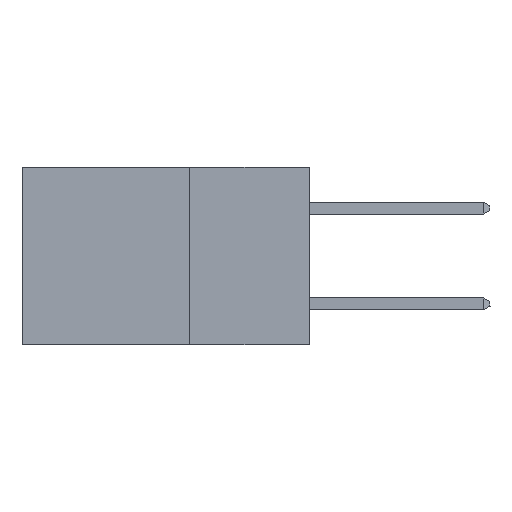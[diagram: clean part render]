
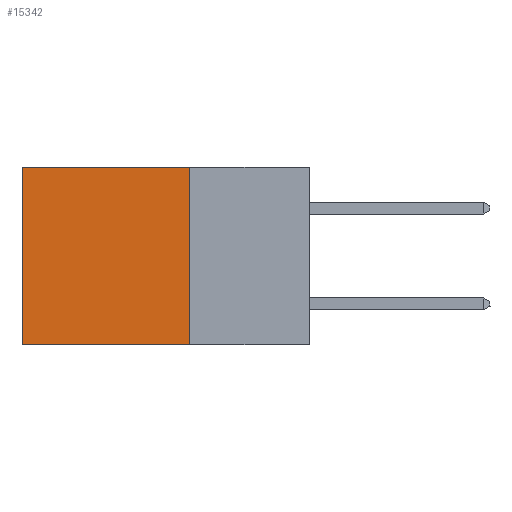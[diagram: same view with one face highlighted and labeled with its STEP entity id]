
A CAD part, left-side view. The second image highlights one B-rep face of the part: STEP entity #15342.
In plain terms, the highlighted planar face has unit normal (-1, 0, 0).
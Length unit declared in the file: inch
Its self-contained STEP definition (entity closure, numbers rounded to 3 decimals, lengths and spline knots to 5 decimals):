
#981 = EDGE_LOOP ( 'NONE', ( #32184, #5134, #12946, #16790 ) ) ;
#1453 = CARTESIAN_POINT ( 'NONE',  ( 0.2875, 0.25, 0. ) ) ;
#1958 = DIRECTION ( 'NONE',  ( 0., 1., 0. ) ) ;
#2166 = CARTESIAN_POINT ( 'NONE',  ( 0.2875, 0.6, 0. ) ) ;
#4519 = CARTESIAN_POINT ( 'NONE',  ( 0.2875, 0.25, -0.37 ) ) ;
#5134 = ORIENTED_EDGE ( 'NONE', *, *, #17647, .F. ) ;
#7228 = DIRECTION ( 'NONE',  ( 0., 1., 0. ) ) ;
#8086 = LINE ( 'NONE', #29395, #22522 ) ;
#8481 = CARTESIAN_POINT ( 'NONE',  ( 0.2875, 0.25, -0.37 ) ) ;
#9485 = DIRECTION ( 'NONE',  ( 1., 0., 0. ) ) ;
#9919 = VERTEX_POINT ( 'NONE', #8481 ) ;
#10377 = EDGE_CURVE ( 'NONE', #26459, #28459, #15561, .T. ) ;
#10738 = VECTOR ( 'NONE', #7228, 39.37008 ) ;
#12946 = ORIENTED_EDGE ( 'NONE', *, *, #13457, .F. ) ;
#13107 = CARTESIAN_POINT ( 'NONE',  ( 0.2875, 0.6, 0. ) ) ;
#13457 = EDGE_CURVE ( 'NONE', #22661, #9919, #8086, .T. ) ;
#14481 = AXIS2_PLACEMENT_3D ( 'NONE', #28485, #9485, #31669 ) ;
#15342 = ADVANCED_FACE ( 'NONE', ( #26312 ), #20982, .F. ) ;
#15561 = LINE ( 'NONE', #13107, #25340 ) ;
#15913 = DIRECTION ( 'NONE',  ( 0., 0., -1. ) ) ;
#16790 = ORIENTED_EDGE ( 'NONE', *, *, #18406, .T. ) ;
#17647 = EDGE_CURVE ( 'NONE', #9919, #28459, #17717, .T. ) ;
#17717 = LINE ( 'NONE', #4519, #10738 ) ;
#17727 = LINE ( 'NONE', #29637, #32180 ) ;
#18406 = EDGE_CURVE ( 'NONE', #22661, #26459, #17727, .T. ) ;
#20982 = PLANE ( 'NONE',  #14481 ) ;
#21791 = DIRECTION ( 'NONE',  ( 0., 0., -1. ) ) ;
#22522 = VECTOR ( 'NONE', #21791, 39.37008 ) ;
#22661 = VERTEX_POINT ( 'NONE', #1453 ) ;
#25340 = VECTOR ( 'NONE', #15913, 39.37008 ) ;
#26312 = FACE_OUTER_BOUND ( 'NONE', #981, .T. ) ;
#26459 = VERTEX_POINT ( 'NONE', #2166 ) ;
#28459 = VERTEX_POINT ( 'NONE', #30521 ) ;
#28485 = CARTESIAN_POINT ( 'NONE',  ( 0.2875, 0.25, 0. ) ) ;
#29395 = CARTESIAN_POINT ( 'NONE',  ( 0.2875, 0.25, 0. ) ) ;
#29637 = CARTESIAN_POINT ( 'NONE',  ( 0.2875, 0.25, 0. ) ) ;
#30521 = CARTESIAN_POINT ( 'NONE',  ( 0.2875, 0.6, -0.37 ) ) ;
#31669 = DIRECTION ( 'NONE',  ( 0., 0., -1. ) ) ;
#32180 = VECTOR ( 'NONE', #1958, 39.37008 ) ;
#32184 = ORIENTED_EDGE ( 'NONE', *, *, #10377, .T. ) ;
